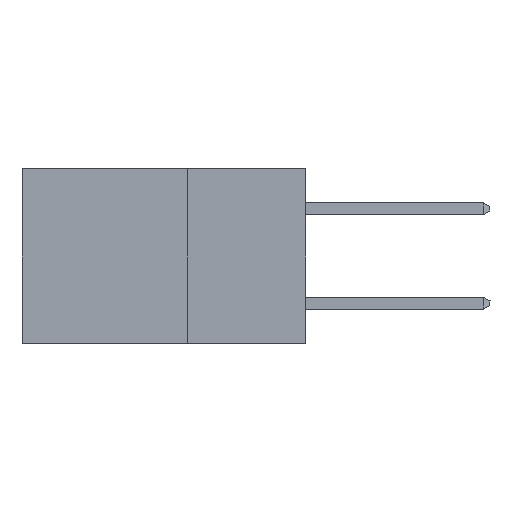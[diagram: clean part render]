
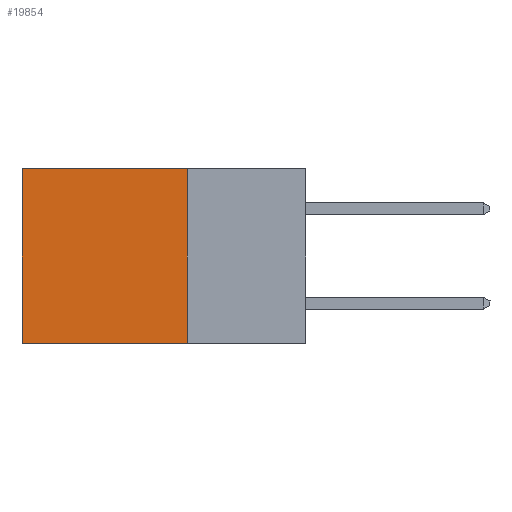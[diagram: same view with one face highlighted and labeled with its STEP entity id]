
A CAD part, left-side view. The second image highlights one B-rep face of the part: STEP entity #19854.
In plain terms, the highlighted planar face has unit normal (-1, 0, 0).
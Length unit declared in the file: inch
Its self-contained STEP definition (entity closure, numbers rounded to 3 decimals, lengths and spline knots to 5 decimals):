
#170 = EDGE_CURVE ( 'NONE', #4202, #18404, #22586, .T. ) ;
#210 = DIRECTION ( 'NONE',  ( 0., 0., -1. ) ) ;
#306 = CARTESIAN_POINT ( 'NONE',  ( 0.2615, 0.6, -0.37 ) ) ;
#1919 = CARTESIAN_POINT ( 'NONE',  ( 0.2615, 0.25, -0.37 ) ) ;
#2401 = LINE ( 'NONE', #6824, #22115 ) ;
#2637 = LINE ( 'NONE', #1919, #7660 ) ;
#3491 = ORIENTED_EDGE ( 'NONE', *, *, #14139, .T. ) ;
#4202 = VERTEX_POINT ( 'NONE', #8620 ) ;
#6824 = CARTESIAN_POINT ( 'NONE',  ( 0.2615, 0.25, -0.37 ) ) ;
#7660 = VECTOR ( 'NONE', #13110, 39.37008 ) ;
#7914 = ORIENTED_EDGE ( 'NONE', *, *, #170, .T. ) ;
#8226 = VECTOR ( 'NONE', #14182, 39.37008 ) ;
#8620 = CARTESIAN_POINT ( 'NONE',  ( 0.2615, 0.6, 0. ) ) ;
#9091 = DIRECTION ( 'NONE',  ( 0., 0., -1. ) ) ;
#11963 = CARTESIAN_POINT ( 'NONE',  ( 0.2615, 0.25, -0.37 ) ) ;
#12353 = CARTESIAN_POINT ( 'NONE',  ( 0.2615, 0.25, 0. ) ) ;
#12850 = VECTOR ( 'NONE', #210, 39.37008 ) ;
#13110 = DIRECTION ( 'NONE',  ( 0., 0., -1. ) ) ;
#14139 = EDGE_CURVE ( 'NONE', #23763, #4202, #18082, .T. ) ;
#14182 = DIRECTION ( 'NONE',  ( 0., 1., 0. ) ) ;
#14719 = AXIS2_PLACEMENT_3D ( 'NONE', #18296, #20116, #9091 ) ;
#15581 = EDGE_CURVE ( 'NONE', #23441, #18404, #2401, .T. ) ;
#16132 = CARTESIAN_POINT ( 'NONE',  ( 0.2615, 0.6, -0.37 ) ) ;
#16466 = PLANE ( 'NONE',  #14719 ) ;
#16749 = EDGE_CURVE ( 'NONE', #23763, #23441, #2637, .T. ) ;
#17943 = FACE_OUTER_BOUND ( 'NONE', #20469, .T. ) ;
#18082 = LINE ( 'NONE', #12353, #8226 ) ;
#18296 = CARTESIAN_POINT ( 'NONE',  ( 0.2615, 0.25, -0.37 ) ) ;
#18404 = VERTEX_POINT ( 'NONE', #16132 ) ;
#18489 = CARTESIAN_POINT ( 'NONE',  ( 0.2615, 0.25, 0. ) ) ;
#19604 = ORIENTED_EDGE ( 'NONE', *, *, #15581, .F. ) ;
#19766 = DIRECTION ( 'NONE',  ( 0., 1., 0. ) ) ;
#19854 = ADVANCED_FACE ( 'NONE', ( #17943 ), #16466, .F. ) ;
#20040 = ORIENTED_EDGE ( 'NONE', *, *, #16749, .F. ) ;
#20116 = DIRECTION ( 'NONE',  ( 1., 0., 0. ) ) ;
#20469 = EDGE_LOOP ( 'NONE', ( #7914, #19604, #20040, #3491 ) ) ;
#22115 = VECTOR ( 'NONE', #19766, 39.37008 ) ;
#22586 = LINE ( 'NONE', #306, #12850 ) ;
#23441 = VERTEX_POINT ( 'NONE', #11963 ) ;
#23763 = VERTEX_POINT ( 'NONE', #18489 ) ;
